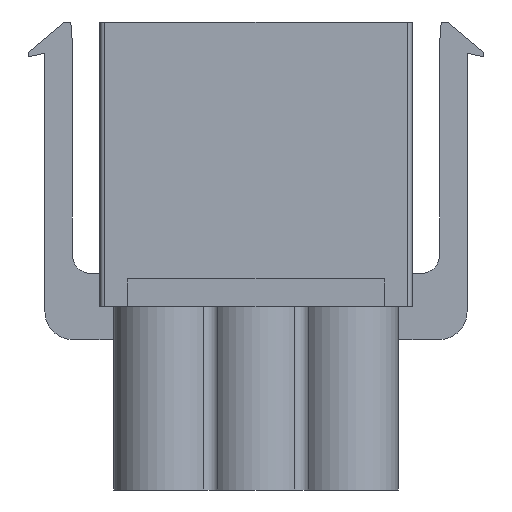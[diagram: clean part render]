
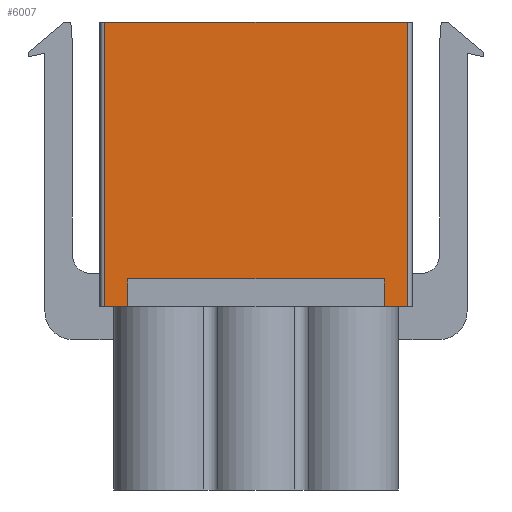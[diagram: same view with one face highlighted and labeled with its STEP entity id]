
A CAD part, front view. The second image highlights one B-rep face of the part: STEP entity #6007.
In plain terms, the highlighted planar face has unit normal (0, -1, 0).
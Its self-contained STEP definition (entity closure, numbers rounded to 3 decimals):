
#19 = EDGE_CURVE ( 'NONE', #1129, #16658, #12794, .T. ) ;
#26 = VERTEX_POINT ( 'NONE', #6316 ) ;
#59 = CARTESIAN_POINT ( 'NONE',  ( 7., -7., -14. ) ) ;
#114 = CARTESIAN_POINT ( 'NONE',  ( -8.25, -7., 0. ) ) ;
#222 = DIRECTION ( 'NONE',  ( 0., 0., 1. ) ) ;
#330 = EDGE_CURVE ( 'NONE', #26, #11031, #2280, .T. ) ;
#491 = ORIENTED_EDGE ( 'NONE', *, *, #2046, .T. ) ;
#668 = CARTESIAN_POINT ( 'NONE',  ( -7., -7., -15.5 ) ) ;
#814 = LINE ( 'NONE', #5994, #11939 ) ;
#1042 = CARTESIAN_POINT ( 'NONE',  ( -7., -7., -14. ) ) ;
#1129 = VERTEX_POINT ( 'NONE', #114 ) ;
#1334 = CARTESIAN_POINT ( 'NONE',  ( 7., -7., -15.5 ) ) ;
#1408 = LINE ( 'NONE', #7776, #3881 ) ;
#2046 = EDGE_CURVE ( 'NONE', #1129, #26, #814, .T. ) ;
#2238 = DIRECTION ( 'NONE',  ( 1., 0., 0. ) ) ;
#2280 = LINE ( 'NONE', #14021, #9741 ) ;
#2391 = VERTEX_POINT ( 'NONE', #1042 ) ;
#3556 = LINE ( 'NONE', #8737, #13130 ) ;
#3596 = ORIENTED_EDGE ( 'NONE', *, *, #330, .T. ) ;
#3791 = FACE_OUTER_BOUND ( 'NONE', #14687, .T. ) ;
#3879 = VERTEX_POINT ( 'NONE', #6313 ) ;
#3881 = VECTOR ( 'NONE', #222, 1000. ) ;
#5071 = DIRECTION ( 'NONE',  ( 0., 0., -1. ) ) ;
#5819 = ORIENTED_EDGE ( 'NONE', *, *, #9409, .F. ) ;
#5994 = CARTESIAN_POINT ( 'NONE',  ( -8.25, -7., -15.5 ) ) ;
#6007 = ADVANCED_FACE ( 'NONE', ( #3791 ), #15785, .T. ) ;
#6096 = EDGE_CURVE ( 'NONE', #3879, #16658, #1408, .T. ) ;
#6313 = CARTESIAN_POINT ( 'NONE',  ( 8.25, -7., -15.5 ) ) ;
#6316 = CARTESIAN_POINT ( 'NONE',  ( -8.25, -7., -15.5 ) ) ;
#6759 = CARTESIAN_POINT ( 'NONE',  ( 7., -7., -14. ) ) ;
#6800 = EDGE_CURVE ( 'NONE', #7392, #2391, #3556, .T. ) ;
#7380 = DIRECTION ( 'NONE',  ( -1., 0., 0. ) ) ;
#7392 = VERTEX_POINT ( 'NONE', #6759 ) ;
#7710 = CARTESIAN_POINT ( 'NONE',  ( 8.25, -7., 0. ) ) ;
#7776 = CARTESIAN_POINT ( 'NONE',  ( 8.25, -7., -15.5 ) ) ;
#8737 = CARTESIAN_POINT ( 'NONE',  ( -7., -7., -14. ) ) ;
#8838 = DIRECTION ( 'NONE',  ( 1., 0., 0. ) ) ;
#9409 = EDGE_CURVE ( 'NONE', #2391, #11031, #16615, .T. ) ;
#9741 = VECTOR ( 'NONE', #16832, 1000. ) ;
#10195 = CARTESIAN_POINT ( 'NONE',  ( -8.5, -7., -15.5 ) ) ;
#10417 = DIRECTION ( 'NONE',  ( 0., 0., -1. ) ) ;
#10505 = CARTESIAN_POINT ( 'NONE',  ( -8.5, -7., -15.5 ) ) ;
#10594 = DIRECTION ( 'NONE',  ( 0., -1., 0. ) ) ;
#10956 = ORIENTED_EDGE ( 'NONE', *, *, #16600, .T. ) ;
#11019 = VECTOR ( 'NONE', #12447, 1000. ) ;
#11031 = VERTEX_POINT ( 'NONE', #668 ) ;
#11460 = ORIENTED_EDGE ( 'NONE', *, *, #6800, .F. ) ;
#11939 = VECTOR ( 'NONE', #15101, 1000. ) ;
#12447 = DIRECTION ( 'NONE',  ( 0., 0., -1. ) ) ;
#12794 = LINE ( 'NONE', #13735, #13003 ) ;
#12851 = AXIS2_PLACEMENT_3D ( 'NONE', #10505, #10594, #10417 ) ;
#12892 = VECTOR ( 'NONE', #5071, 1000. ) ;
#13003 = VECTOR ( 'NONE', #2238, 1000. ) ;
#13130 = VECTOR ( 'NONE', #7380, 1000. ) ;
#13484 = EDGE_CURVE ( 'NONE', #14139, #3879, #14196, .T. ) ;
#13735 = CARTESIAN_POINT ( 'NONE',  ( -8.5, -7., 0. ) ) ;
#14021 = CARTESIAN_POINT ( 'NONE',  ( -8.5, -7., -15.5 ) ) ;
#14061 = ORIENTED_EDGE ( 'NONE', *, *, #19, .F. ) ;
#14087 = VECTOR ( 'NONE', #8838, 1000. ) ;
#14139 = VERTEX_POINT ( 'NONE', #1334 ) ;
#14196 = LINE ( 'NONE', #10195, #14087 ) ;
#14687 = EDGE_LOOP ( 'NONE', ( #14061, #491, #3596, #5819, #11460, #10956, #16095, #16422 ) ) ;
#15101 = DIRECTION ( 'NONE',  ( 0., 0., -1. ) ) ;
#15164 = CARTESIAN_POINT ( 'NONE',  ( -7., -7., -14. ) ) ;
#15785 = PLANE ( 'NONE',  #12851 ) ;
#16095 = ORIENTED_EDGE ( 'NONE', *, *, #13484, .T. ) ;
#16422 = ORIENTED_EDGE ( 'NONE', *, *, #6096, .T. ) ;
#16600 = EDGE_CURVE ( 'NONE', #7392, #14139, #16741, .T. ) ;
#16615 = LINE ( 'NONE', #15164, #11019 ) ;
#16658 = VERTEX_POINT ( 'NONE', #7710 ) ;
#16741 = LINE ( 'NONE', #59, #12892 ) ;
#16832 = DIRECTION ( 'NONE',  ( 1., 0., 0. ) ) ;
